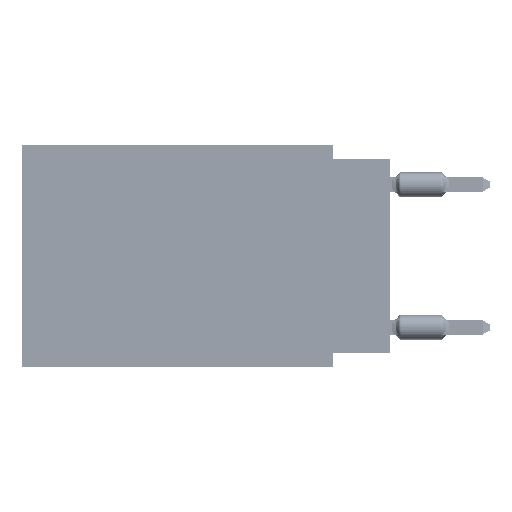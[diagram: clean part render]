
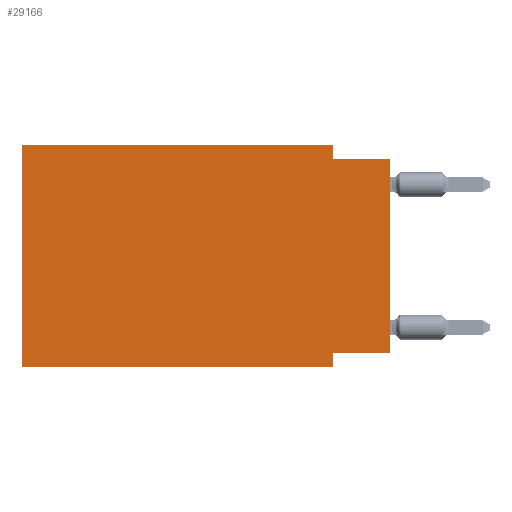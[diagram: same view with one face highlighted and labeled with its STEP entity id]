
A CAD part, left-side view. The second image highlights one B-rep face of the part: STEP entity #29166.
In plain terms, the highlighted planar face has unit normal (-1, 0, 0).
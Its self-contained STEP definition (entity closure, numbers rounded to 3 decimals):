
#521 = ORIENTED_EDGE ( 'NONE', *, *, #47908, .T. ) ;
#569 = VERTEX_POINT ( 'NONE', #62534 ) ;
#2123 = DIRECTION ( 'NONE',  ( 0., 0., 1. ) ) ;
#3404 = CARTESIAN_POINT ( 'NONE',  ( 0., 0., 0. ) ) ;
#7054 = FACE_OUTER_BOUND ( 'NONE', #49064, .T. ) ;
#8646 = EDGE_CURVE ( 'NONE', #17306, #569, #47825, .T. ) ;
#10124 = ORIENTED_EDGE ( 'NONE', *, *, #36771, .F. ) ;
#10432 = ORIENTED_EDGE ( 'NONE', *, *, #42844, .F. ) ;
#10963 = CARTESIAN_POINT ( 'NONE',  ( 0., 2.54, 0. ) ) ;
#11989 = DIRECTION ( 'NONE',  ( 0., -1., 0. ) ) ;
#12194 = VERTEX_POINT ( 'NONE', #23055 ) ;
#12356 = CARTESIAN_POINT ( 'NONE',  ( 0., 0., -0.635 ) ) ;
#13862 = DIRECTION ( 'NONE',  ( 0., 0., -1. ) ) ;
#14310 = CARTESIAN_POINT ( 'NONE',  ( 0., 16.383, -9.906 ) ) ;
#17306 = VERTEX_POINT ( 'NONE', #14310 ) ;
#17566 = VECTOR ( 'NONE', #44531, 1000. ) ;
#18875 = ORIENTED_EDGE ( 'NONE', *, *, #37258, .T. ) ;
#19132 = DIRECTION ( 'NONE',  ( 1., 0., 0. ) ) ;
#19153 = CARTESIAN_POINT ( 'NONE',  ( 0., 16.383, -9.906 ) ) ;
#20788 = LINE ( 'NONE', #3404, #17566 ) ;
#23055 = CARTESIAN_POINT ( 'NONE',  ( 0., 0., -0.635 ) ) ;
#24813 = CARTESIAN_POINT ( 'NONE',  ( 0., 16.383, 0. ) ) ;
#25343 = CARTESIAN_POINT ( 'NONE',  ( 0., 2.54, -9.906 ) ) ;
#25779 = CARTESIAN_POINT ( 'NONE',  ( 0., 0., -9.271 ) ) ;
#26856 = VECTOR ( 'NONE', #11989, 1000. ) ;
#29166 = ADVANCED_FACE ( 'NONE', ( #7054 ), #59887, .F. ) ;
#29853 = CARTESIAN_POINT ( 'NONE',  ( 0., 2.54, -9.271 ) ) ;
#29870 = EDGE_CURVE ( 'NONE', #67503, #47707, #46785, .T. ) ;
#30473 = CARTESIAN_POINT ( 'NONE',  ( 0., 16.383, 0. ) ) ;
#30539 = VECTOR ( 'NONE', #69088, 1000. ) ;
#31319 = CARTESIAN_POINT ( 'NONE',  ( 0., 16.383, 0. ) ) ;
#31593 = CARTESIAN_POINT ( 'NONE',  ( 0., 2.54, -9.906 ) ) ;
#36610 = DIRECTION ( 'NONE',  ( 0., -1., 0. ) ) ;
#36771 = EDGE_CURVE ( 'NONE', #569, #67503, #61103, .T. ) ;
#37258 = EDGE_CURVE ( 'NONE', #17306, #47709, #47840, .T. ) ;
#40033 = VERTEX_POINT ( 'NONE', #71664 ) ;
#40858 = VECTOR ( 'NONE', #42173, 1000. ) ;
#42173 = DIRECTION ( 'NONE',  ( 0., -1., 0. ) ) ;
#42380 = DIRECTION ( 'NONE',  ( 0., 1., 0. ) ) ;
#42844 = EDGE_CURVE ( 'NONE', #47707, #12194, #64053, .T. ) ;
#44530 = ORIENTED_EDGE ( 'NONE', *, *, #61114, .F. ) ;
#44531 = DIRECTION ( 'NONE',  ( 0., 0., 1. ) ) ;
#45185 = ORIENTED_EDGE ( 'NONE', *, *, #29870, .F. ) ;
#46262 = VECTOR ( 'NONE', #13862, 1000. ) ;
#46785 = LINE ( 'NONE', #10963, #30539 ) ;
#46877 = VECTOR ( 'NONE', #2123, 1000. ) ;
#47707 = VERTEX_POINT ( 'NONE', #59309 ) ;
#47709 = VERTEX_POINT ( 'NONE', #25343 ) ;
#47825 = LINE ( 'NONE', #24813, #46877 ) ;
#47840 = LINE ( 'NONE', #19153, #40858 ) ;
#47908 = EDGE_CURVE ( 'NONE', #40033, #12194, #20788, .T. ) ;
#49064 = EDGE_LOOP ( 'NONE', ( #521, #10432, #45185, #10124, #67606, #18875, #52771, #44530 ) ) ;
#49234 = VECTOR ( 'NONE', #36610, 1000. ) ;
#52771 = ORIENTED_EDGE ( 'NONE', *, *, #59132, .F. ) ;
#54885 = VECTOR ( 'NONE', #42380, 1000. ) ;
#58167 = AXIS2_PLACEMENT_3D ( 'NONE', #30473, #19132, #65540 ) ;
#59132 = EDGE_CURVE ( 'NONE', #61423, #47709, #66674, .T. ) ;
#59309 = CARTESIAN_POINT ( 'NONE',  ( 0., 2.54, -0.635 ) ) ;
#59372 = LINE ( 'NONE', #25779, #54885 ) ;
#59887 = PLANE ( 'NONE',  #58167 ) ;
#61103 = LINE ( 'NONE', #31319, #49234 ) ;
#61114 = EDGE_CURVE ( 'NONE', #40033, #61423, #59372, .T. ) ;
#61423 = VERTEX_POINT ( 'NONE', #29853 ) ;
#62534 = CARTESIAN_POINT ( 'NONE',  ( 0., 16.383, 0. ) ) ;
#64053 = LINE ( 'NONE', #12356, #26856 ) ;
#65540 = DIRECTION ( 'NONE',  ( 0., 0., -1. ) ) ;
#66674 = LINE ( 'NONE', #31593, #46262 ) ;
#67503 = VERTEX_POINT ( 'NONE', #72177 ) ;
#67606 = ORIENTED_EDGE ( 'NONE', *, *, #8646, .F. ) ;
#69088 = DIRECTION ( 'NONE',  ( 0., 0., -1. ) ) ;
#71664 = CARTESIAN_POINT ( 'NONE',  ( 0., 0., -9.271 ) ) ;
#72177 = CARTESIAN_POINT ( 'NONE',  ( 0., 2.54, 0. ) ) ;
